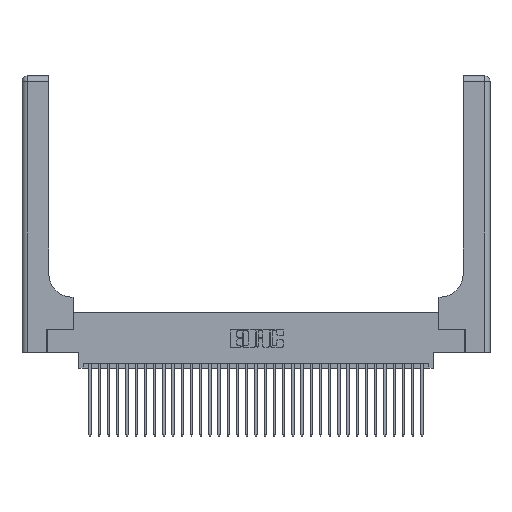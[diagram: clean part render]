
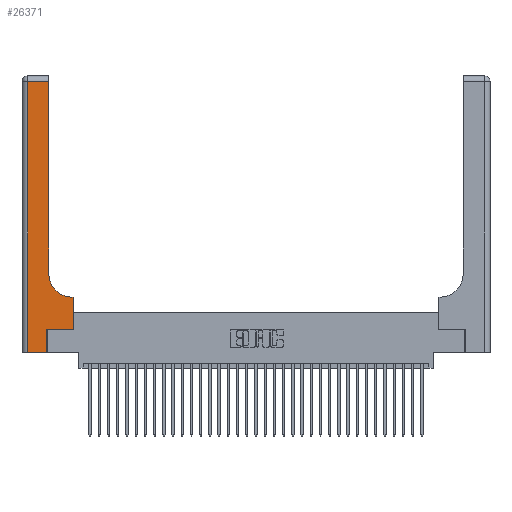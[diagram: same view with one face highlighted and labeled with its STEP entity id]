
A CAD part, top view. The second image highlights one B-rep face of the part: STEP entity #26371.
In plain terms, the highlighted planar face has unit normal (0, 0, 1).
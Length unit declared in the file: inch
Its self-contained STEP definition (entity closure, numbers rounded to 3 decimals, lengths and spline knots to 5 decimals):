
#692 = ORIENTED_EDGE ( 'NONE', *, *, #25504, .T. ) ;
#1136 = VECTOR ( 'NONE', #10929, 39.37008 ) ;
#1730 = EDGE_CURVE ( 'NONE', #10182, #28957, #11741, .T. ) ;
#2299 = CARTESIAN_POINT ( 'NONE',  ( 0., 3., 0.37 ) ) ;
#2620 = DIRECTION ( 'NONE',  ( 1., 0., 0. ) ) ;
#3577 = VECTOR ( 'NONE', #26919, 39.37008 ) ;
#4089 = ORIENTED_EDGE ( 'NONE', *, *, #1730, .T. ) ;
#4658 = EDGE_CURVE ( 'NONE', #5996, #24027, #8528, .T. ) ;
#5044 = DIRECTION ( 'NONE',  ( 0., 0., -1. ) ) ;
#5068 = VERTEX_POINT ( 'NONE', #7338 ) ;
#5753 = CARTESIAN_POINT ( 'NONE',  ( 0.2915, 3., 0.37 ) ) ;
#5898 = VERTEX_POINT ( 'NONE', #17495 ) ;
#5996 = VERTEX_POINT ( 'NONE', #18078 ) ;
#6005 = DIRECTION ( 'NONE',  ( 0., 1., 0. ) ) ;
#6194 = LINE ( 'NONE', #7927, #33273 ) ;
#7338 = CARTESIAN_POINT ( 'NONE',  ( 0.06, 0., 0.37 ) ) ;
#7467 = LINE ( 'NONE', #19120, #1136 ) ;
#7927 = CARTESIAN_POINT ( 'NONE',  ( 0.269, 0.25, 0.37 ) ) ;
#8447 = DIRECTION ( 'NONE',  ( 0., 1., 0. ) ) ;
#8528 = LINE ( 'NONE', #5753, #30172 ) ;
#8765 = AXIS2_PLACEMENT_3D ( 'NONE', #9545, #28538, #12286 ) ;
#9545 = CARTESIAN_POINT ( 'NONE',  ( 0.5415, 0.85, 0.37 ) ) ;
#10182 = VERTEX_POINT ( 'NONE', #29127 ) ;
#10258 = ORIENTED_EDGE ( 'NONE', *, *, #16768, .T. ) ;
#10929 = DIRECTION ( 'NONE',  ( -1., 0., 0. ) ) ;
#11741 = LINE ( 'NONE', #25968, #25337 ) ;
#11833 = VERTEX_POINT ( 'NONE', #31467 ) ;
#12286 = DIRECTION ( 'NONE',  ( 1., 0., 0. ) ) ;
#13877 = VERTEX_POINT ( 'NONE', #18709 ) ;
#14137 = EDGE_LOOP ( 'NONE', ( #33119, #10258, #27712, #692, #4089, #29115, #27014, #18991, #28746 ) ) ;
#15283 = LINE ( 'NONE', #30743, #28854 ) ;
#15443 = AXIS2_PLACEMENT_3D ( 'NONE', #2299, #5044, #24008 ) ;
#16148 = CARTESIAN_POINT ( 'NONE',  ( 0.06, 3., 0.37 ) ) ;
#16286 = CARTESIAN_POINT ( 'NONE',  ( 0.2915, 2.94, 0.37 ) ) ;
#16768 = EDGE_CURVE ( 'NONE', #24027, #11833, #28202, .T. ) ;
#16949 = VERTEX_POINT ( 'NONE', #21896 ) ;
#17495 = CARTESIAN_POINT ( 'NONE',  ( 0.5585, 0.6, 0.37 ) ) ;
#18078 = CARTESIAN_POINT ( 'NONE',  ( 0.2915, 0.85, 0.37 ) ) ;
#18709 = CARTESIAN_POINT ( 'NONE',  ( 0.5585, 0.25, 0.37 ) ) ;
#18991 = ORIENTED_EDGE ( 'NONE', *, *, #32614, .T. ) ;
#19120 = CARTESIAN_POINT ( 'NONE',  ( 0.2915, 0.6, 0.37 ) ) ;
#20132 = VECTOR ( 'NONE', #26629, 39.37008 ) ;
#21896 = CARTESIAN_POINT ( 'NONE',  ( 0.5415, 0.6, 0.37 ) ) ;
#22129 = CIRCLE ( 'NONE', #8765, 0.25 ) ;
#23090 = EDGE_CURVE ( 'NONE', #16949, #5996, #22129, .T. ) ;
#23912 = CARTESIAN_POINT ( 'NONE',  ( 0., 2.94, 0.37 ) ) ;
#24008 = DIRECTION ( 'NONE',  ( -1., 0., 0. ) ) ;
#24027 = VERTEX_POINT ( 'NONE', #16286 ) ;
#24972 = CARTESIAN_POINT ( 'NONE',  ( 0.5585, 0.25, 0.37 ) ) ;
#25227 = LINE ( 'NONE', #16148, #3577 ) ;
#25337 = VECTOR ( 'NONE', #28683, 39.37008 ) ;
#25504 = EDGE_CURVE ( 'NONE', #5068, #10182, #15283, .T. ) ;
#25968 = CARTESIAN_POINT ( 'NONE',  ( 0.269, 0., 0.37 ) ) ;
#26371 = ADVANCED_FACE ( 'NONE', ( #34683 ), #34719, .F. ) ;
#26415 = VECTOR ( 'NONE', #6005, 39.37008 ) ;
#26629 = DIRECTION ( 'NONE',  ( -1., 0., 0. ) ) ;
#26919 = DIRECTION ( 'NONE',  ( 0., -1., 0. ) ) ;
#27014 = ORIENTED_EDGE ( 'NONE', *, *, #30645, .T. ) ;
#27288 = LINE ( 'NONE', #24972, #26415 ) ;
#27712 = ORIENTED_EDGE ( 'NONE', *, *, #28907, .T. ) ;
#28202 = LINE ( 'NONE', #23912, #20132 ) ;
#28538 = DIRECTION ( 'NONE',  ( 0., 0., -1. ) ) ;
#28683 = DIRECTION ( 'NONE',  ( 0., 1., 0. ) ) ;
#28746 = ORIENTED_EDGE ( 'NONE', *, *, #23090, .T. ) ;
#28854 = VECTOR ( 'NONE', #33431, 39.37008 ) ;
#28907 = EDGE_CURVE ( 'NONE', #11833, #5068, #25227, .T. ) ;
#28957 = VERTEX_POINT ( 'NONE', #31990 ) ;
#29054 = EDGE_CURVE ( 'NONE', #28957, #13877, #6194, .T. ) ;
#29115 = ORIENTED_EDGE ( 'NONE', *, *, #29054, .T. ) ;
#29127 = CARTESIAN_POINT ( 'NONE',  ( 0.269, 0., 0.37 ) ) ;
#30172 = VECTOR ( 'NONE', #8447, 39.37008 ) ;
#30645 = EDGE_CURVE ( 'NONE', #13877, #5898, #27288, .T. ) ;
#30743 = CARTESIAN_POINT ( 'NONE',  ( 0., 0., 0.37 ) ) ;
#31467 = CARTESIAN_POINT ( 'NONE',  ( 0.06, 2.94, 0.37 ) ) ;
#31990 = CARTESIAN_POINT ( 'NONE',  ( 0.269, 0.25, 0.37 ) ) ;
#32614 = EDGE_CURVE ( 'NONE', #5898, #16949, #7467, .T. ) ;
#33119 = ORIENTED_EDGE ( 'NONE', *, *, #4658, .T. ) ;
#33273 = VECTOR ( 'NONE', #2620, 39.37008 ) ;
#33431 = DIRECTION ( 'NONE',  ( 1., 0., 0. ) ) ;
#34683 = FACE_OUTER_BOUND ( 'NONE', #14137, .T. ) ;
#34719 = PLANE ( 'NONE',  #15443 ) ;
